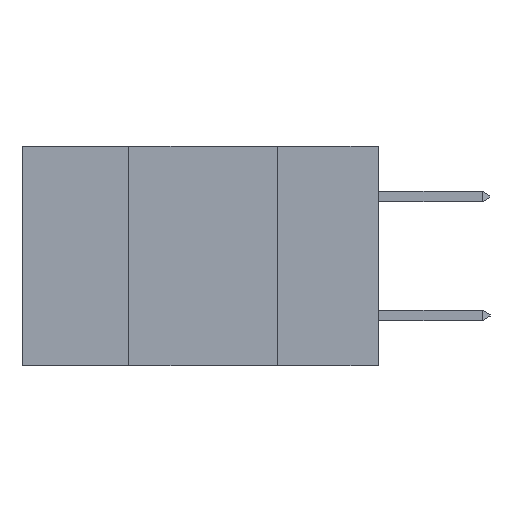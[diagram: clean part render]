
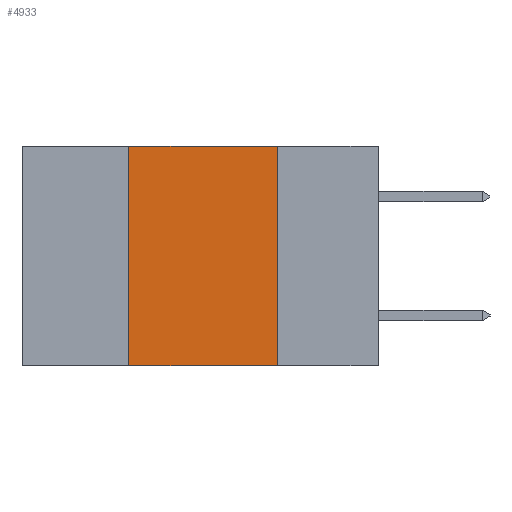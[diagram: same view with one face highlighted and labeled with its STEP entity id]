
A CAD part, left-side view. The second image highlights one B-rep face of the part: STEP entity #4933.
In plain terms, the highlighted planar face has unit normal (-1, 0, 0).
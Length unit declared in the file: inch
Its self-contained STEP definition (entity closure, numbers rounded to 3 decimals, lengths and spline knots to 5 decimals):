
#451 = ORIENTED_EDGE ( 'NONE', *, *, #4405, .T. ) ;
#632 = DIRECTION ( 'NONE',  ( 0., 0., -1. ) ) ;
#638 = ORIENTED_EDGE ( 'NONE', *, *, #4451, .F. ) ;
#737 = CARTESIAN_POINT ( 'NONE',  ( 0., 0.17, -0.37 ) ) ;
#1081 = CARTESIAN_POINT ( 'NONE',  ( 0., 0.6, 0. ) ) ;
#1184 = DIRECTION ( 'NONE',  ( 1., 0., 0. ) ) ;
#1262 = DIRECTION ( 'NONE',  ( 0., 0., -1. ) ) ;
#2292 = PLANE ( 'NONE',  #9408 ) ;
#2471 = EDGE_LOOP ( 'NONE', ( #8691, #9094, #638, #451 ) ) ;
#2680 = LINE ( 'NONE', #10769, #8697 ) ;
#3959 = CARTESIAN_POINT ( 'NONE',  ( 0., 0.42, -0.37 ) ) ;
#4327 = LINE ( 'NONE', #12477, #12359 ) ;
#4405 = EDGE_CURVE ( 'NONE', #5700, #5533, #4735, .T. ) ;
#4451 = EDGE_CURVE ( 'NONE', #5700, #12516, #4327, .T. ) ;
#4498 = EDGE_CURVE ( 'NONE', #12516, #4502, #2680, .T. ) ;
#4502 = VERTEX_POINT ( 'NONE', #10291 ) ;
#4735 = LINE ( 'NONE', #14324, #10497 ) ;
#4778 = EDGE_CURVE ( 'NONE', #4502, #5533, #6447, .T. ) ;
#4933 = ADVANCED_FACE ( 'NONE', ( #5904 ), #2292, .F. ) ;
#5533 = VERTEX_POINT ( 'NONE', #13240 ) ;
#5700 = VERTEX_POINT ( 'NONE', #3959 ) ;
#5904 = FACE_OUTER_BOUND ( 'NONE', #2471, .T. ) ;
#6096 = VECTOR ( 'NONE', #632, 39.37008 ) ;
#6447 = LINE ( 'NONE', #737, #6096 ) ;
#7628 = CARTESIAN_POINT ( 'NONE',  ( 0., 0.42, 0. ) ) ;
#8691 = ORIENTED_EDGE ( 'NONE', *, *, #4778, .F. ) ;
#8697 = VECTOR ( 'NONE', #11181, 39.37008 ) ;
#9094 = ORIENTED_EDGE ( 'NONE', *, *, #4498, .F. ) ;
#9408 = AXIS2_PLACEMENT_3D ( 'NONE', #1081, #1184, #1262 ) ;
#10291 = CARTESIAN_POINT ( 'NONE',  ( 0., 0.17, 0. ) ) ;
#10497 = VECTOR ( 'NONE', #14061, 39.37008 ) ;
#10769 = CARTESIAN_POINT ( 'NONE',  ( 0., 0.6, 0. ) ) ;
#11181 = DIRECTION ( 'NONE',  ( 0., -1., 0. ) ) ;
#12212 = DIRECTION ( 'NONE',  ( 0., 0., 1. ) ) ;
#12359 = VECTOR ( 'NONE', #12212, 39.37008 ) ;
#12477 = CARTESIAN_POINT ( 'NONE',  ( 0., 0.42, -0.37 ) ) ;
#12516 = VERTEX_POINT ( 'NONE', #7628 ) ;
#13240 = CARTESIAN_POINT ( 'NONE',  ( 0., 0.17, -0.37 ) ) ;
#14061 = DIRECTION ( 'NONE',  ( 0., -1., 0. ) ) ;
#14324 = CARTESIAN_POINT ( 'NONE',  ( 0., 0.6, -0.37 ) ) ;
